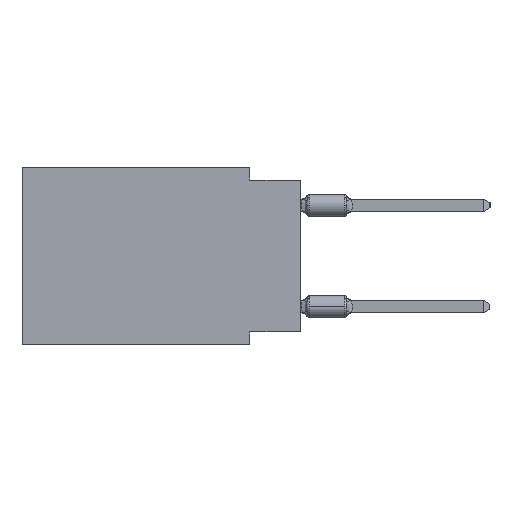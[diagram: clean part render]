
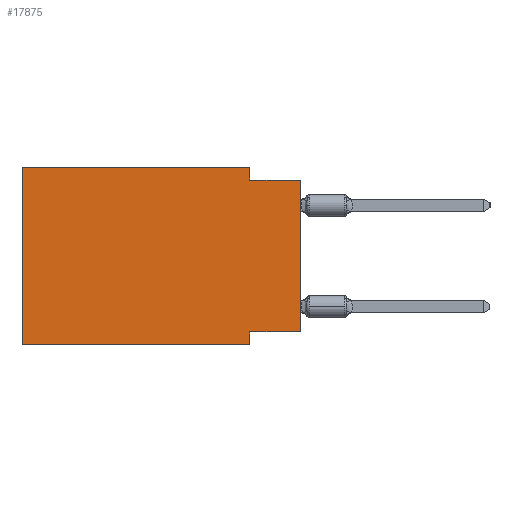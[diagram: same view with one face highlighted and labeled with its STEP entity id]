
A CAD part, left-side view. The second image highlights one B-rep face of the part: STEP entity #17875.
In plain terms, the highlighted planar face has unit normal (-1, 0, 0).
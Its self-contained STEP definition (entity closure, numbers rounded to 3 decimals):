
#950 = EDGE_CURVE ( 'NONE', #37214, #44115, #27621, .T. ) ;
#1129 = LINE ( 'NONE', #32977, #49575 ) ;
#1657 = LINE ( 'NONE', #50458, #8672 ) ;
#2230 = ORIENTED_EDGE ( 'NONE', *, *, #9479, .F. ) ;
#4064 = CARTESIAN_POINT ( 'NONE',  ( 0., 2.54, -8.255 ) ) ;
#4660 = EDGE_CURVE ( 'NONE', #34618, #7227, #1129, .T. ) ;
#5002 = DIRECTION ( 'NONE',  ( 0., -1., 0. ) ) ;
#6389 = LINE ( 'NONE', #19808, #9475 ) ;
#6662 = DIRECTION ( 'NONE',  ( 0., 0., 1. ) ) ;
#7227 = VERTEX_POINT ( 'NONE', #21450 ) ;
#8672 = VECTOR ( 'NONE', #19482, 1000. ) ;
#8854 = EDGE_CURVE ( 'NONE', #57255, #47174, #6389, .T. ) ;
#9475 = VECTOR ( 'NONE', #6662, 1000. ) ;
#9479 = EDGE_CURVE ( 'NONE', #7227, #55466, #17322, .T. ) ;
#10529 = EDGE_CURVE ( 'NONE', #56961, #34618, #41979, .T. ) ;
#11475 = EDGE_CURVE ( 'NONE', #56961, #44115, #45047, .T. ) ;
#11537 = PLANE ( 'NONE',  #57645 ) ;
#12146 = DIRECTION ( 'NONE',  ( 0., 0., -1. ) ) ;
#14009 = ORIENTED_EDGE ( 'NONE', *, *, #11475, .T. ) ;
#14466 = EDGE_CURVE ( 'NONE', #55466, #47174, #1657, .T. ) ;
#16902 = DIRECTION ( 'NONE',  ( 0., 0., -1. ) ) ;
#17197 = EDGE_LOOP ( 'NONE', ( #25779, #35833, #2230, #47820, #45715, #14009, #50627, #45266 ) ) ;
#17322 = LINE ( 'NONE', #35167, #27265 ) ;
#17875 = ADVANCED_FACE ( 'NONE', ( #52192 ), #11537, .F. ) ;
#19417 = EDGE_CURVE ( 'NONE', #57255, #37214, #51305, .T. ) ;
#19482 = DIRECTION ( 'NONE',  ( 0., -1., 0. ) ) ;
#19808 = CARTESIAN_POINT ( 'NONE',  ( 0., 0., 0. ) ) ;
#20628 = CARTESIAN_POINT ( 'NONE',  ( 0., 2.54, -8.89 ) ) ;
#21450 = CARTESIAN_POINT ( 'NONE',  ( 0., 2.54, 0. ) ) ;
#24439 = CARTESIAN_POINT ( 'NONE',  ( 0., 13.97, 0. ) ) ;
#24479 = CARTESIAN_POINT ( 'NONE',  ( 0., 13.97, -8.89 ) ) ;
#25300 = DIRECTION ( 'NONE',  ( 1., 0., 0. ) ) ;
#25779 = ORIENTED_EDGE ( 'NONE', *, *, #8854, .T. ) ;
#27265 = VECTOR ( 'NONE', #52992, 1000. ) ;
#27621 = LINE ( 'NONE', #44085, #37195 ) ;
#28101 = CARTESIAN_POINT ( 'NONE',  ( 0., 13.97, -8.89 ) ) ;
#28218 = DIRECTION ( 'NONE',  ( 0., 1., 0. ) ) ;
#29790 = VECTOR ( 'NONE', #28218, 1000. ) ;
#30101 = CARTESIAN_POINT ( 'NONE',  ( 0., 2.54, -0.635 ) ) ;
#32977 = CARTESIAN_POINT ( 'NONE',  ( 0., 13.97, 0. ) ) ;
#33167 = CARTESIAN_POINT ( 'NONE',  ( 0., 0., -8.255 ) ) ;
#34618 = VERTEX_POINT ( 'NONE', #37145 ) ;
#35167 = CARTESIAN_POINT ( 'NONE',  ( 0., 2.54, 0. ) ) ;
#35833 = ORIENTED_EDGE ( 'NONE', *, *, #14466, .F. ) ;
#36037 = CARTESIAN_POINT ( 'NONE',  ( 0., 0., -0.635 ) ) ;
#37145 = CARTESIAN_POINT ( 'NONE',  ( 0., 13.97, 0. ) ) ;
#37195 = VECTOR ( 'NONE', #16902, 1000. ) ;
#37214 = VERTEX_POINT ( 'NONE', #4064 ) ;
#41979 = LINE ( 'NONE', #24439, #48793 ) ;
#44085 = CARTESIAN_POINT ( 'NONE',  ( 0., 2.54, -8.89 ) ) ;
#44115 = VERTEX_POINT ( 'NONE', #20628 ) ;
#45047 = LINE ( 'NONE', #28101, #55570 ) ;
#45266 = ORIENTED_EDGE ( 'NONE', *, *, #19417, .F. ) ;
#45715 = ORIENTED_EDGE ( 'NONE', *, *, #10529, .F. ) ;
#47174 = VERTEX_POINT ( 'NONE', #36037 ) ;
#47820 = ORIENTED_EDGE ( 'NONE', *, *, #4660, .F. ) ;
#48793 = VECTOR ( 'NONE', #55409, 1000. ) ;
#49575 = VECTOR ( 'NONE', #50532, 1000. ) ;
#50432 = CARTESIAN_POINT ( 'NONE',  ( 0., 0., -8.255 ) ) ;
#50458 = CARTESIAN_POINT ( 'NONE',  ( 0., 0., -0.635 ) ) ;
#50532 = DIRECTION ( 'NONE',  ( 0., -1., 0. ) ) ;
#50627 = ORIENTED_EDGE ( 'NONE', *, *, #950, .F. ) ;
#51305 = LINE ( 'NONE', #33167, #29790 ) ;
#52192 = FACE_OUTER_BOUND ( 'NONE', #17197, .T. ) ;
#52992 = DIRECTION ( 'NONE',  ( 0., 0., -1. ) ) ;
#55409 = DIRECTION ( 'NONE',  ( 0., 0., 1. ) ) ;
#55466 = VERTEX_POINT ( 'NONE', #30101 ) ;
#55570 = VECTOR ( 'NONE', #5002, 1000. ) ;
#56268 = CARTESIAN_POINT ( 'NONE',  ( 0., 13.97, 0. ) ) ;
#56961 = VERTEX_POINT ( 'NONE', #24479 ) ;
#57255 = VERTEX_POINT ( 'NONE', #50432 ) ;
#57645 = AXIS2_PLACEMENT_3D ( 'NONE', #56268, #25300, #12146 ) ;
